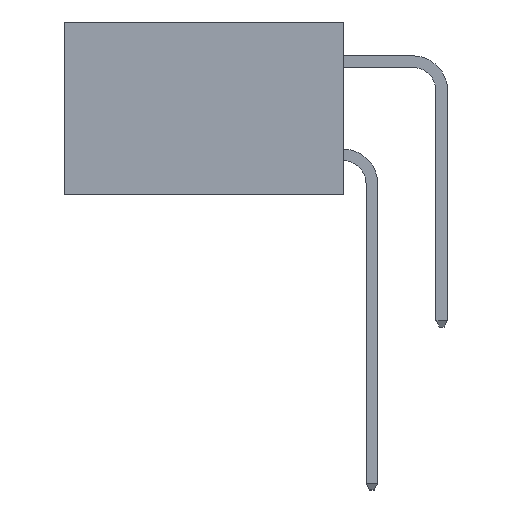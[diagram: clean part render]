
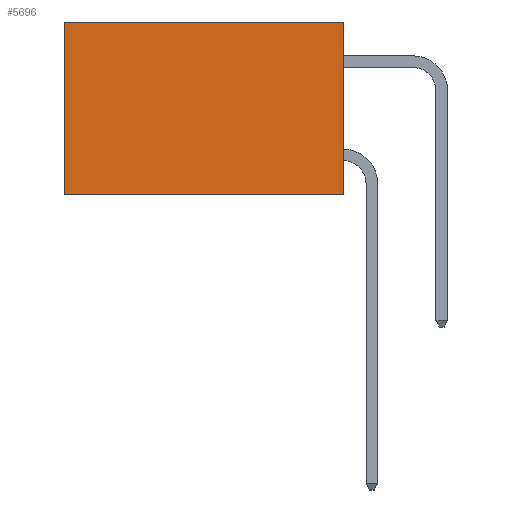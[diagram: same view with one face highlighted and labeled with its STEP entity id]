
A CAD part, left-side view. The second image highlights one B-rep face of the part: STEP entity #5696.
In plain terms, the highlighted planar face has unit normal (-1, 0, 0).
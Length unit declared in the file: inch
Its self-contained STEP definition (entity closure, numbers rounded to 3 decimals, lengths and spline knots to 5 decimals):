
#1 = EDGE_CURVE ( 'NONE', #12440, #935, #6772, .T. ) ;
#306 = ORIENTED_EDGE ( 'NONE', *, *, #1, .T. ) ;
#601 = CARTESIAN_POINT ( 'NONE',  ( 0.2615, 0., -0.37 ) ) ;
#666 = ORIENTED_EDGE ( 'NONE', *, *, #1968, .F. ) ;
#935 = VERTEX_POINT ( 'NONE', #7613 ) ;
#1497 = VERTEX_POINT ( 'NONE', #3032 ) ;
#1731 = FACE_OUTER_BOUND ( 'NONE', #2149, .T. ) ;
#1741 = DIRECTION ( 'NONE',  ( 1., 0., 0. ) ) ;
#1811 = LINE ( 'NONE', #8554, #9580 ) ;
#1933 = LINE ( 'NONE', #3967, #9389 ) ;
#1968 = EDGE_CURVE ( 'NONE', #5809, #935, #1811, .T. ) ;
#2149 = EDGE_LOOP ( 'NONE', ( #306, #666, #4545, #6358 ) ) ;
#2910 = DIRECTION ( 'NONE',  ( 0., 1., 0. ) ) ;
#2939 = DIRECTION ( 'NONE',  ( 0., 1., 0. ) ) ;
#3032 = CARTESIAN_POINT ( 'NONE',  ( 0.2615, 0., 0. ) ) ;
#3967 = CARTESIAN_POINT ( 'NONE',  ( 0.2615, 0., 0. ) ) ;
#4206 = VECTOR ( 'NONE', #7106, 39.37008 ) ;
#4408 = VECTOR ( 'NONE', #8996, 39.37008 ) ;
#4545 = ORIENTED_EDGE ( 'NONE', *, *, #11222, .F. ) ;
#5205 = AXIS2_PLACEMENT_3D ( 'NONE', #601, #1741, #8578 ) ;
#5696 = ADVANCED_FACE ( 'NONE', ( #1731 ), #6774, .F. ) ;
#5809 = VERTEX_POINT ( 'NONE', #9665 ) ;
#6333 = CARTESIAN_POINT ( 'NONE',  ( 0.2615, 0.6, 0. ) ) ;
#6358 = ORIENTED_EDGE ( 'NONE', *, *, #11956, .T. ) ;
#6772 = LINE ( 'NONE', #10830, #4206 ) ;
#6774 = PLANE ( 'NONE',  #5205 ) ;
#7106 = DIRECTION ( 'NONE',  ( 0., 0., -1. ) ) ;
#7228 = LINE ( 'NONE', #9967, #4408 ) ;
#7613 = CARTESIAN_POINT ( 'NONE',  ( 0.2615, 0.6, -0.37 ) ) ;
#8554 = CARTESIAN_POINT ( 'NONE',  ( 0.2615, 0., -0.37 ) ) ;
#8578 = DIRECTION ( 'NONE',  ( 0., 0., -1. ) ) ;
#8996 = DIRECTION ( 'NONE',  ( 0., 0., -1. ) ) ;
#9389 = VECTOR ( 'NONE', #2939, 39.37008 ) ;
#9580 = VECTOR ( 'NONE', #2910, 39.37008 ) ;
#9665 = CARTESIAN_POINT ( 'NONE',  ( 0.2615, 0., -0.37 ) ) ;
#9967 = CARTESIAN_POINT ( 'NONE',  ( 0.2615, 0., -0.37 ) ) ;
#10830 = CARTESIAN_POINT ( 'NONE',  ( 0.2615, 0.6, -0.37 ) ) ;
#11222 = EDGE_CURVE ( 'NONE', #1497, #5809, #7228, .T. ) ;
#11956 = EDGE_CURVE ( 'NONE', #1497, #12440, #1933, .T. ) ;
#12440 = VERTEX_POINT ( 'NONE', #6333 ) ;
